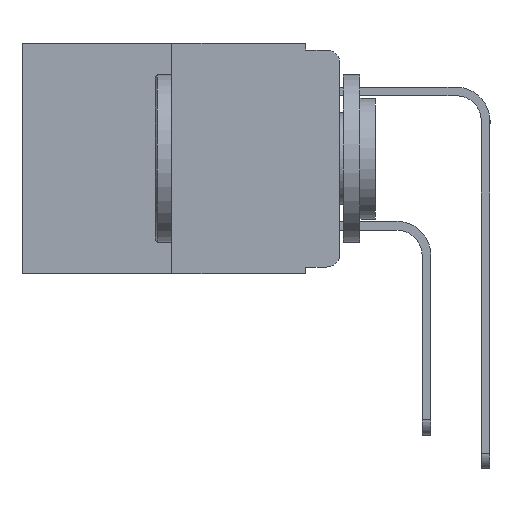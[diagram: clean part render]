
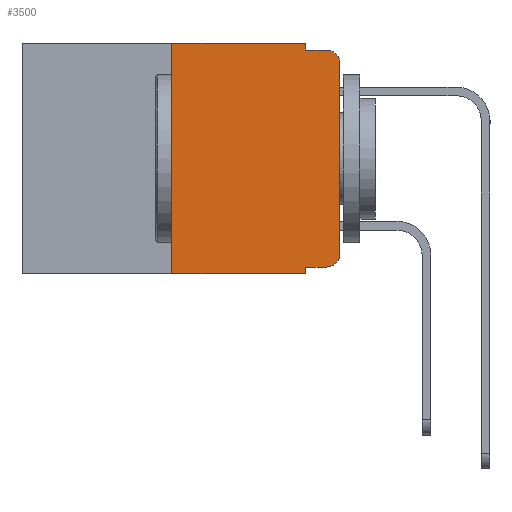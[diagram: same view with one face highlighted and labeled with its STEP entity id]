
A CAD part, left-side view. The second image highlights one B-rep face of the part: STEP entity #3500.
In plain terms, the highlighted planar face has unit normal (-1, 0, 0).
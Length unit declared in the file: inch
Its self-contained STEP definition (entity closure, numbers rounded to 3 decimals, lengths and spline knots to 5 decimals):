
#508 = EDGE_CURVE ( 'NONE', #1852, #8332, #14306, .T. ) ;
#617 = CIRCLE ( 'NONE', #7266, 0.02 ) ;
#817 = CARTESIAN_POINT ( 'NONE',  ( 0., 0.473, -0.343 ) ) ;
#1554 = DIRECTION ( 'NONE',  ( 0., -1., 0. ) ) ;
#1832 = ORIENTED_EDGE ( 'NONE', *, *, #17855, .F. ) ;
#1852 = VERTEX_POINT ( 'NONE', #20199 ) ;
#2151 = ORIENTED_EDGE ( 'NONE', *, *, #11263, .T. ) ;
#2792 = DIRECTION ( 'NONE',  ( 0., 0., 1. ) ) ;
#2964 = DIRECTION ( 'NONE',  ( 0., 0., -1. ) ) ;
#3102 = DIRECTION ( 'NONE',  ( 0., -1., 0. ) ) ;
#3270 = CARTESIAN_POINT ( 'NONE',  ( 0., 0., -0.03 ) ) ;
#3500 = ADVANCED_FACE ( 'NONE', ( #3746 ), #11933, .F. ) ;
#3746 = FACE_OUTER_BOUND ( 'NONE', #21665, .T. ) ;
#3757 = VERTEX_POINT ( 'NONE', #10768 ) ;
#3958 = VERTEX_POINT ( 'NONE', #9709 ) ;
#3993 = VECTOR ( 'NONE', #2964, 39.37008 ) ;
#4206 = EDGE_CURVE ( 'NONE', #20996, #16025, #17799, .T. ) ;
#4491 = EDGE_CURVE ( 'NONE', #16088, #14474, #8094, .T. ) ;
#4556 = VECTOR ( 'NONE', #8279, 39.37008 ) ;
#4896 = CARTESIAN_POINT ( 'NONE',  ( 0., 0.051, -0.01 ) ) ;
#5327 = VECTOR ( 'NONE', #1554, 39.37008 ) ;
#5686 = VECTOR ( 'NONE', #3102, 39.37008 ) ;
#6334 = CARTESIAN_POINT ( 'NONE',  ( 0., 0.473, 0. ) ) ;
#6953 = CARTESIAN_POINT ( 'NONE',  ( 0., 0.02, -0.313 ) ) ;
#7266 = AXIS2_PLACEMENT_3D ( 'NONE', #6953, #19346, #8853 ) ;
#7629 = VECTOR ( 'NONE', #2792, 39.37008 ) ;
#7714 = VECTOR ( 'NONE', #20335, 39.37008 ) ;
#8094 = CIRCLE ( 'NONE', #21318, 0.02 ) ;
#8279 = DIRECTION ( 'NONE',  ( 0., 0., 1. ) ) ;
#8296 = CARTESIAN_POINT ( 'NONE',  ( 0., 0., 0. ) ) ;
#8327 = DIRECTION ( 'NONE',  ( 1., 0., 0. ) ) ;
#8332 = VERTEX_POINT ( 'NONE', #21973 ) ;
#8633 = CARTESIAN_POINT ( 'NONE',  ( 0., 0.051, -0.333 ) ) ;
#8853 = DIRECTION ( 'NONE',  ( 0., 0., -1. ) ) ;
#9709 = CARTESIAN_POINT ( 'NONE',  ( 0., 0.051, -0.343 ) ) ;
#10057 = ORIENTED_EDGE ( 'NONE', *, *, #15178, .F. ) ;
#10506 = EDGE_CURVE ( 'NONE', #15955, #14222, #16139, .T. ) ;
#10514 = DIRECTION ( 'NONE',  ( 0., -1., 0. ) ) ;
#10768 = CARTESIAN_POINT ( 'NONE',  ( 0., 0., -0.313 ) ) ;
#11057 = AXIS2_PLACEMENT_3D ( 'NONE', #6334, #8327, #20576 ) ;
#11236 = EDGE_CURVE ( 'NONE', #16025, #14474, #15298, .T. ) ;
#11263 = EDGE_CURVE ( 'NONE', #14222, #3757, #617, .T. ) ;
#11278 = DIRECTION ( 'NONE',  ( -1., 0., 0. ) ) ;
#11757 = CARTESIAN_POINT ( 'NONE',  ( 0., 0.051, 0. ) ) ;
#11884 = CARTESIAN_POINT ( 'NONE',  ( 0., 0.02, -0.01 ) ) ;
#11933 = PLANE ( 'NONE',  #11057 ) ;
#12021 = ORIENTED_EDGE ( 'NONE', *, *, #18734, .T. ) ;
#12085 = VECTOR ( 'NONE', #10514, 39.37008 ) ;
#12341 = CARTESIAN_POINT ( 'NONE',  ( 0., 0.051, -0.01 ) ) ;
#13112 = ORIENTED_EDGE ( 'NONE', *, *, #4206, .F. ) ;
#13780 = DIRECTION ( 'NONE',  ( 0., -1., 0. ) ) ;
#13979 = CARTESIAN_POINT ( 'NONE',  ( 0., 0.051, 0. ) ) ;
#14222 = VERTEX_POINT ( 'NONE', #18033 ) ;
#14306 = LINE ( 'NONE', #20530, #4556 ) ;
#14474 = VERTEX_POINT ( 'NONE', #11884 ) ;
#15178 = EDGE_CURVE ( 'NONE', #15955, #3958, #21173, .T. ) ;
#15298 = LINE ( 'NONE', #12341, #5686 ) ;
#15516 = ORIENTED_EDGE ( 'NONE', *, *, #11236, .F. ) ;
#15955 = VERTEX_POINT ( 'NONE', #20745 ) ;
#16025 = VERTEX_POINT ( 'NONE', #4896 ) ;
#16088 = VERTEX_POINT ( 'NONE', #3270 ) ;
#16139 = LINE ( 'NONE', #8633, #12085 ) ;
#16331 = ORIENTED_EDGE ( 'NONE', *, *, #508, .F. ) ;
#17064 = LINE ( 'NONE', #8296, #7629 ) ;
#17799 = LINE ( 'NONE', #13979, #3993 ) ;
#17855 = EDGE_CURVE ( 'NONE', #8332, #20996, #23080, .T. ) ;
#18033 = CARTESIAN_POINT ( 'NONE',  ( 0., 0.02, -0.333 ) ) ;
#18435 = VECTOR ( 'NONE', #13780, 39.37008 ) ;
#18725 = ORIENTED_EDGE ( 'NONE', *, *, #19014, .T. ) ;
#18734 = EDGE_CURVE ( 'NONE', #1852, #3958, #23033, .T. ) ;
#19014 = EDGE_CURVE ( 'NONE', #3757, #16088, #17064, .T. ) ;
#19346 = DIRECTION ( 'NONE',  ( -1., 0., 0. ) ) ;
#19841 = ORIENTED_EDGE ( 'NONE', *, *, #10506, .T. ) ;
#20199 = CARTESIAN_POINT ( 'NONE',  ( 0., 0.25, -0.343 ) ) ;
#20335 = DIRECTION ( 'NONE',  ( 0., 0., -1. ) ) ;
#20530 = CARTESIAN_POINT ( 'NONE',  ( 0., 0.25, 0. ) ) ;
#20576 = DIRECTION ( 'NONE',  ( 0., 0., -1. ) ) ;
#20745 = CARTESIAN_POINT ( 'NONE',  ( 0., 0.051, -0.333 ) ) ;
#20988 = CARTESIAN_POINT ( 'NONE',  ( 0., 0.051, 0. ) ) ;
#20996 = VERTEX_POINT ( 'NONE', #20988 ) ;
#21173 = LINE ( 'NONE', #11757, #7714 ) ;
#21318 = AXIS2_PLACEMENT_3D ( 'NONE', #21603, #11278, #23374 ) ;
#21603 = CARTESIAN_POINT ( 'NONE',  ( 0., 0.02, -0.03 ) ) ;
#21665 = EDGE_LOOP ( 'NONE', ( #18725, #21958, #15516, #13112, #1832, #16331, #12021, #10057, #19841, #2151 ) ) ;
#21958 = ORIENTED_EDGE ( 'NONE', *, *, #4491, .T. ) ;
#21973 = CARTESIAN_POINT ( 'NONE',  ( 0., 0.25, 0. ) ) ;
#23001 = CARTESIAN_POINT ( 'NONE',  ( 0., 0.473, 0. ) ) ;
#23033 = LINE ( 'NONE', #817, #18435 ) ;
#23080 = LINE ( 'NONE', #23001, #5327 ) ;
#23374 = DIRECTION ( 'NONE',  ( 0., 0., -1. ) ) ;
